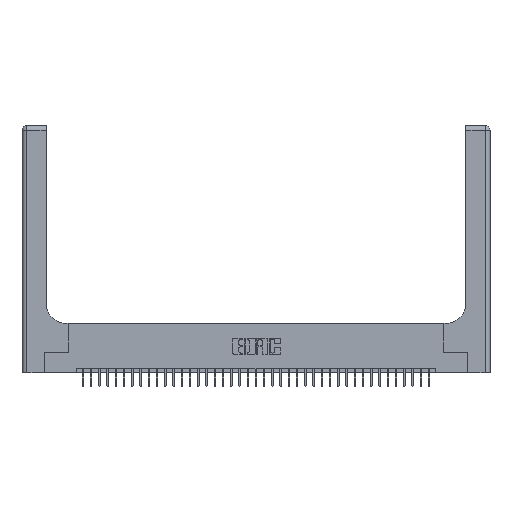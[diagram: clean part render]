
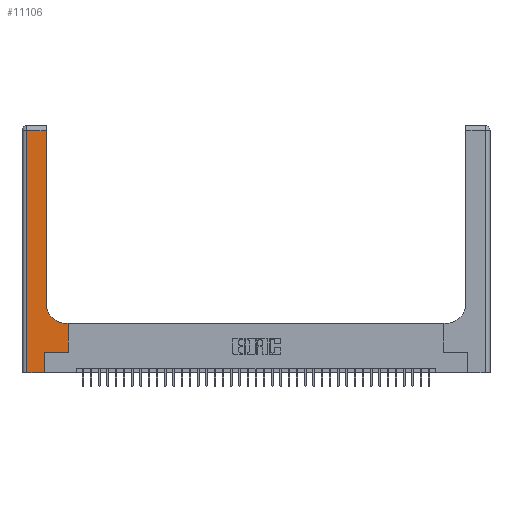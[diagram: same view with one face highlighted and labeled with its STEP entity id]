
A CAD part, top view. The second image highlights one B-rep face of the part: STEP entity #11106.
In plain terms, the highlighted planar face has unit normal (0, 0, 1).
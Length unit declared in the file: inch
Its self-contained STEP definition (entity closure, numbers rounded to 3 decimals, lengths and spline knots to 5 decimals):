
#457 = VECTOR ( 'NONE', #7899, 39.37008 ) ;
#487 = DIRECTION ( 'NONE',  ( -1., 0., 0. ) ) ;
#1393 = LINE ( 'NONE', #4856, #457 ) ;
#2136 = VECTOR ( 'NONE', #12783, 39.37008 ) ;
#3087 = CARTESIAN_POINT ( 'NONE',  ( 0., 0., 0.37 ) ) ;
#3413 = CARTESIAN_POINT ( 'NONE',  ( 0.2915, 0.85, 0.37 ) ) ;
#3763 = EDGE_CURVE ( 'NONE', #24848, #17022, #36037, .T. ) ;
#4856 = CARTESIAN_POINT ( 'NONE',  ( 0.5585, 0.25, 0.37 ) ) ;
#5649 = AXIS2_PLACEMENT_3D ( 'NONE', #31967, #13985, #34940 ) ;
#6337 = CARTESIAN_POINT ( 'NONE',  ( 0., 2.94, 0.37 ) ) ;
#7385 = EDGE_LOOP ( 'NONE', ( #33664, #14286, #18338, #31029, #25798, #21145, #37790, #36820, #16342 ) ) ;
#7521 = EDGE_CURVE ( 'NONE', #28401, #36588, #11829, .T. ) ;
#7599 = CARTESIAN_POINT ( 'NONE',  ( 0.5585, 0.6, 0.37 ) ) ;
#7771 = CARTESIAN_POINT ( 'NONE',  ( 0.269, 0.25, 0.37 ) ) ;
#7899 = DIRECTION ( 'NONE',  ( 0., 1., 0. ) ) ;
#9753 = CARTESIAN_POINT ( 'NONE',  ( 0.06, 3., 0.37 ) ) ;
#9900 = VECTOR ( 'NONE', #16605, 39.37008 ) ;
#10184 = DIRECTION ( 'NONE',  ( 0., 1., 0. ) ) ;
#11106 = ADVANCED_FACE ( 'NONE', ( #15663 ), #12523, .F. ) ;
#11201 = LINE ( 'NONE', #16093, #33282 ) ;
#11618 = CARTESIAN_POINT ( 'NONE',  ( 0.2915, 2.94, 0.37 ) ) ;
#11829 = CIRCLE ( 'NONE', #5649, 0.25 ) ;
#12357 = CARTESIAN_POINT ( 'NONE',  ( 0.269, 0., 0.37 ) ) ;
#12426 = CARTESIAN_POINT ( 'NONE',  ( 0.06, 2.94, 0.37 ) ) ;
#12499 = DIRECTION ( 'NONE',  ( 1., 0., 0. ) ) ;
#12523 = PLANE ( 'NONE',  #24840 ) ;
#12783 = DIRECTION ( 'NONE',  ( 0., -1., 0. ) ) ;
#13064 = VECTOR ( 'NONE', #36321, 39.37008 ) ;
#13353 = VERTEX_POINT ( 'NONE', #11618 ) ;
#13985 = DIRECTION ( 'NONE',  ( 0., 0., -1. ) ) ;
#14286 = ORIENTED_EDGE ( 'NONE', *, *, #31149, .T. ) ;
#15663 = FACE_OUTER_BOUND ( 'NONE', #7385, .T. ) ;
#16093 = CARTESIAN_POINT ( 'NONE',  ( 0.2915, 3., 0.37 ) ) ;
#16104 = CARTESIAN_POINT ( 'NONE',  ( 0.269, 0., 0.37 ) ) ;
#16342 = ORIENTED_EDGE ( 'NONE', *, *, #7521, .T. ) ;
#16410 = VERTEX_POINT ( 'NONE', #23328 ) ;
#16605 = DIRECTION ( 'NONE',  ( -1., 0., 0. ) ) ;
#17022 = VERTEX_POINT ( 'NONE', #7771 ) ;
#18338 = ORIENTED_EDGE ( 'NONE', *, *, #35186, .T. ) ;
#18544 = DIRECTION ( 'NONE',  ( 0., 0., -1. ) ) ;
#19923 = EDGE_CURVE ( 'NONE', #17022, #16410, #30492, .T. ) ;
#20698 = LINE ( 'NONE', #37423, #9900 ) ;
#21145 = ORIENTED_EDGE ( 'NONE', *, *, #19923, .T. ) ;
#21809 = LINE ( 'NONE', #6337, #28863 ) ;
#23265 = LINE ( 'NONE', #3087, #30333 ) ;
#23328 = CARTESIAN_POINT ( 'NONE',  ( 0.5585, 0.25, 0.37 ) ) ;
#24840 = AXIS2_PLACEMENT_3D ( 'NONE', #33523, #18544, #487 ) ;
#24848 = VERTEX_POINT ( 'NONE', #16104 ) ;
#25798 = ORIENTED_EDGE ( 'NONE', *, *, #3763, .T. ) ;
#26208 = LINE ( 'NONE', #9753, #2136 ) ;
#26251 = VERTEX_POINT ( 'NONE', #28624 ) ;
#27355 = CARTESIAN_POINT ( 'NONE',  ( 0.269, 0.25, 0.37 ) ) ;
#28401 = VERTEX_POINT ( 'NONE', #35910 ) ;
#28624 = CARTESIAN_POINT ( 'NONE',  ( 0.06, 0., 0.37 ) ) ;
#28863 = VECTOR ( 'NONE', #30428, 39.37008 ) ;
#29541 = VECTOR ( 'NONE', #12499, 39.37008 ) ;
#30220 = DIRECTION ( 'NONE',  ( 1., 0., 0. ) ) ;
#30333 = VECTOR ( 'NONE', #30220, 39.37008 ) ;
#30428 = DIRECTION ( 'NONE',  ( -1., 0., 0. ) ) ;
#30448 = EDGE_CURVE ( 'NONE', #26251, #24848, #23265, .T. ) ;
#30492 = LINE ( 'NONE', #27355, #29541 ) ;
#31029 = ORIENTED_EDGE ( 'NONE', *, *, #30448, .T. ) ;
#31149 = EDGE_CURVE ( 'NONE', #13353, #38528, #21809, .T. ) ;
#31967 = CARTESIAN_POINT ( 'NONE',  ( 0.5415, 0.85, 0.37 ) ) ;
#32920 = EDGE_CURVE ( 'NONE', #16410, #35373, #1393, .T. ) ;
#33282 = VECTOR ( 'NONE', #10184, 39.37008 ) ;
#33523 = CARTESIAN_POINT ( 'NONE',  ( 0., 3., 0.37 ) ) ;
#33664 = ORIENTED_EDGE ( 'NONE', *, *, #34729, .T. ) ;
#34729 = EDGE_CURVE ( 'NONE', #36588, #13353, #11201, .T. ) ;
#34940 = DIRECTION ( 'NONE',  ( 1., 0., 0. ) ) ;
#35186 = EDGE_CURVE ( 'NONE', #38528, #26251, #26208, .T. ) ;
#35373 = VERTEX_POINT ( 'NONE', #7599 ) ;
#35910 = CARTESIAN_POINT ( 'NONE',  ( 0.5415, 0.6, 0.37 ) ) ;
#36037 = LINE ( 'NONE', #12357, #13064 ) ;
#36321 = DIRECTION ( 'NONE',  ( 0., 1., 0. ) ) ;
#36588 = VERTEX_POINT ( 'NONE', #3413 ) ;
#36797 = EDGE_CURVE ( 'NONE', #35373, #28401, #20698, .T. ) ;
#36820 = ORIENTED_EDGE ( 'NONE', *, *, #36797, .T. ) ;
#37423 = CARTESIAN_POINT ( 'NONE',  ( 0.2915, 0.6, 0.37 ) ) ;
#37790 = ORIENTED_EDGE ( 'NONE', *, *, #32920, .T. ) ;
#38528 = VERTEX_POINT ( 'NONE', #12426 ) ;
